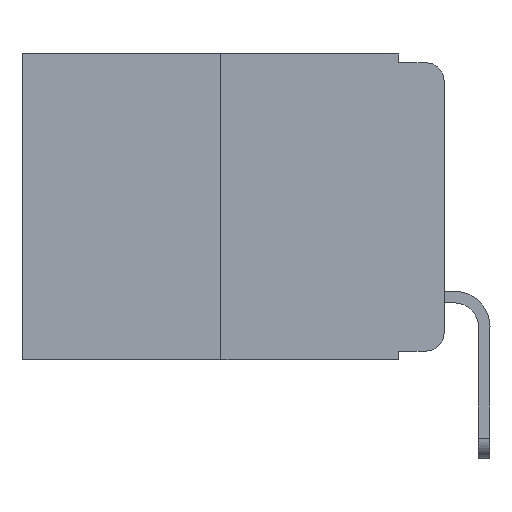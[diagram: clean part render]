
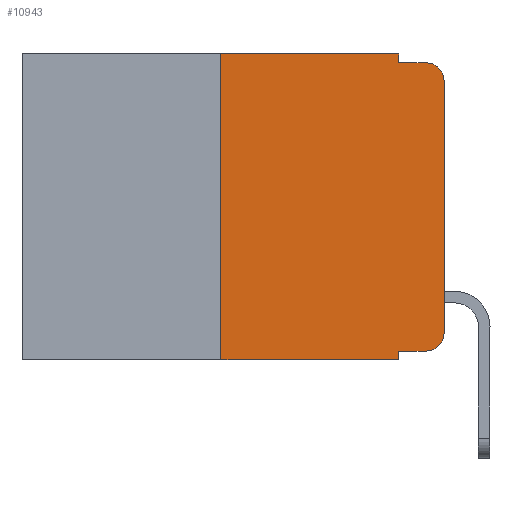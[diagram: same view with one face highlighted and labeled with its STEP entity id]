
A CAD part, left-side view. The second image highlights one B-rep face of the part: STEP entity #10943.
In plain terms, the highlighted planar face has unit normal (-1, 0, 0).
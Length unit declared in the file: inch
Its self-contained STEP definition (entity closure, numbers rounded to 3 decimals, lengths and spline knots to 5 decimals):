
#281 = ORIENTED_EDGE ( 'NONE', *, *, #22417, .T. ) ;
#1246 = CARTESIAN_POINT ( 'NONE',  ( 0., 0., -0.03 ) ) ;
#1555 = EDGE_CURVE ( 'NONE', #2160, #10083, #20709, .T. ) ;
#1633 = CARTESIAN_POINT ( 'NONE',  ( 0., 0.02, -0.01 ) ) ;
#1858 = EDGE_CURVE ( 'NONE', #10207, #8363, #13165, .T. ) ;
#2160 = VERTEX_POINT ( 'NONE', #4646 ) ;
#2235 = EDGE_CURVE ( 'NONE', #21852, #10207, #2972, .T. ) ;
#2405 = CARTESIAN_POINT ( 'NONE',  ( 0., 0.02, -0.313 ) ) ;
#2720 = LINE ( 'NONE', #11357, #7240 ) ;
#2832 = LINE ( 'NONE', #8519, #21076 ) ;
#2972 = LINE ( 'NONE', #3197, #12522 ) ;
#3197 = CARTESIAN_POINT ( 'NONE',  ( 0., 0.051, 0. ) ) ;
#3759 = EDGE_CURVE ( 'NONE', #5604, #21852, #18507, .T. ) ;
#4428 = DIRECTION ( 'NONE',  ( 0., 0., -1. ) ) ;
#4646 = CARTESIAN_POINT ( 'NONE',  ( 0., 0., -0.313 ) ) ;
#4695 = DIRECTION ( 'NONE',  ( -1., 0., 0. ) ) ;
#5202 = ORIENTED_EDGE ( 'NONE', *, *, #13688, .F. ) ;
#5240 = CARTESIAN_POINT ( 'NONE',  ( 0., 0.473, 0. ) ) ;
#5485 = CARTESIAN_POINT ( 'NONE',  ( 0., 0.473, -0.343 ) ) ;
#5604 = VERTEX_POINT ( 'NONE', #12452 ) ;
#5707 = VECTOR ( 'NONE', #14690, 39.37008 ) ;
#5912 = CIRCLE ( 'NONE', #21047, 0.02 ) ;
#6110 = CARTESIAN_POINT ( 'NONE',  ( 0., 0.02, -0.333 ) ) ;
#7240 = VECTOR ( 'NONE', #15205, 39.37008 ) ;
#7349 = DIRECTION ( 'NONE',  ( 0., -1., 0. ) ) ;
#7648 = EDGE_CURVE ( 'NONE', #18903, #2160, #5912, .T. ) ;
#8055 = CARTESIAN_POINT ( 'NONE',  ( 0., 0.051, 0. ) ) ;
#8334 = CARTESIAN_POINT ( 'NONE',  ( 0., 0.051, -0.333 ) ) ;
#8363 = VERTEX_POINT ( 'NONE', #1633 ) ;
#8519 = CARTESIAN_POINT ( 'NONE',  ( 0., 0.25, 0. ) ) ;
#8936 = EDGE_LOOP ( 'NONE', ( #21253, #281, #20917, #23751, #20757, #20871, #12370, #5202, #9599, #16803 ) ) ;
#9242 = EDGE_CURVE ( 'NONE', #23481, #24066, #10676, .T. ) ;
#9300 = CARTESIAN_POINT ( 'NONE',  ( 0., 0.051, -0.01 ) ) ;
#9359 = DIRECTION ( 'NONE',  ( 1., 0., 0. ) ) ;
#9599 = ORIENTED_EDGE ( 'NONE', *, *, #23267, .T. ) ;
#9971 = DIRECTION ( 'NONE',  ( -1., 0., 0. ) ) ;
#10083 = VERTEX_POINT ( 'NONE', #1246 ) ;
#10093 = CARTESIAN_POINT ( 'NONE',  ( 0., 0.051, -0.343 ) ) ;
#10207 = VERTEX_POINT ( 'NONE', #14569 ) ;
#10308 = VECTOR ( 'NONE', #15790, 39.37008 ) ;
#10676 = LINE ( 'NONE', #5485, #11253 ) ;
#10943 = ADVANCED_FACE ( 'NONE', ( #21744 ), #11150, .F. ) ;
#11150 = PLANE ( 'NONE',  #21237 ) ;
#11253 = VECTOR ( 'NONE', #18634, 39.37008 ) ;
#11357 = CARTESIAN_POINT ( 'NONE',  ( 0., 0.051, -0.333 ) ) ;
#11892 = DIRECTION ( 'NONE',  ( 0., 0., -1. ) ) ;
#12270 = CARTESIAN_POINT ( 'NONE',  ( 0., 0.02, -0.03 ) ) ;
#12370 = ORIENTED_EDGE ( 'NONE', *, *, #9242, .T. ) ;
#12398 = EDGE_CURVE ( 'NONE', #23481, #5604, #2832, .T. ) ;
#12452 = CARTESIAN_POINT ( 'NONE',  ( 0., 0.25, 0. ) ) ;
#12522 = VECTOR ( 'NONE', #20522, 39.37008 ) ;
#13165 = LINE ( 'NONE', #9300, #5707 ) ;
#13688 = EDGE_CURVE ( 'NONE', #21162, #24066, #15045, .T. ) ;
#14295 = CARTESIAN_POINT ( 'NONE',  ( 0., 0.051, 0. ) ) ;
#14569 = CARTESIAN_POINT ( 'NONE',  ( 0., 0.051, -0.01 ) ) ;
#14690 = DIRECTION ( 'NONE',  ( 0., -1., 0. ) ) ;
#15045 = LINE ( 'NONE', #8055, #10308 ) ;
#15205 = DIRECTION ( 'NONE',  ( 0., -1., 0. ) ) ;
#15557 = VECTOR ( 'NONE', #17423, 39.37008 ) ;
#15781 = VECTOR ( 'NONE', #7349, 39.37008 ) ;
#15790 = DIRECTION ( 'NONE',  ( 0., 0., -1. ) ) ;
#16094 = CARTESIAN_POINT ( 'NONE',  ( 0., 0.25, -0.343 ) ) ;
#16803 = ORIENTED_EDGE ( 'NONE', *, *, #7648, .T. ) ;
#17345 = CARTESIAN_POINT ( 'NONE',  ( 0., 0., 0. ) ) ;
#17368 = AXIS2_PLACEMENT_3D ( 'NONE', #12270, #4695, #4428 ) ;
#17423 = DIRECTION ( 'NONE',  ( 0., 0., 1. ) ) ;
#18380 = DIRECTION ( 'NONE',  ( 0., 0., 1. ) ) ;
#18507 = LINE ( 'NONE', #5240, #15781 ) ;
#18634 = DIRECTION ( 'NONE',  ( 0., -1., 0. ) ) ;
#18903 = VERTEX_POINT ( 'NONE', #6110 ) ;
#20522 = DIRECTION ( 'NONE',  ( 0., 0., -1. ) ) ;
#20709 = LINE ( 'NONE', #17345, #15557 ) ;
#20757 = ORIENTED_EDGE ( 'NONE', *, *, #3759, .F. ) ;
#20871 = ORIENTED_EDGE ( 'NONE', *, *, #12398, .F. ) ;
#20917 = ORIENTED_EDGE ( 'NONE', *, *, #1858, .F. ) ;
#21047 = AXIS2_PLACEMENT_3D ( 'NONE', #2405, #9971, #11892 ) ;
#21076 = VECTOR ( 'NONE', #18380, 39.37008 ) ;
#21162 = VERTEX_POINT ( 'NONE', #8334 ) ;
#21237 = AXIS2_PLACEMENT_3D ( 'NONE', #24532, #9359, #24625 ) ;
#21253 = ORIENTED_EDGE ( 'NONE', *, *, #1555, .T. ) ;
#21611 = CIRCLE ( 'NONE', #17368, 0.02 ) ;
#21744 = FACE_OUTER_BOUND ( 'NONE', #8936, .T. ) ;
#21852 = VERTEX_POINT ( 'NONE', #14295 ) ;
#22417 = EDGE_CURVE ( 'NONE', #10083, #8363, #21611, .T. ) ;
#23267 = EDGE_CURVE ( 'NONE', #21162, #18903, #2720, .T. ) ;
#23481 = VERTEX_POINT ( 'NONE', #16094 ) ;
#23751 = ORIENTED_EDGE ( 'NONE', *, *, #2235, .F. ) ;
#24066 = VERTEX_POINT ( 'NONE', #10093 ) ;
#24532 = CARTESIAN_POINT ( 'NONE',  ( 0., 0.473, 0. ) ) ;
#24625 = DIRECTION ( 'NONE',  ( 0., 0., -1. ) ) ;
